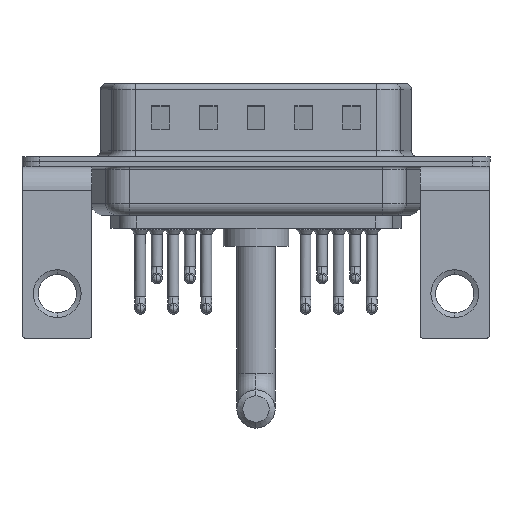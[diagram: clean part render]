
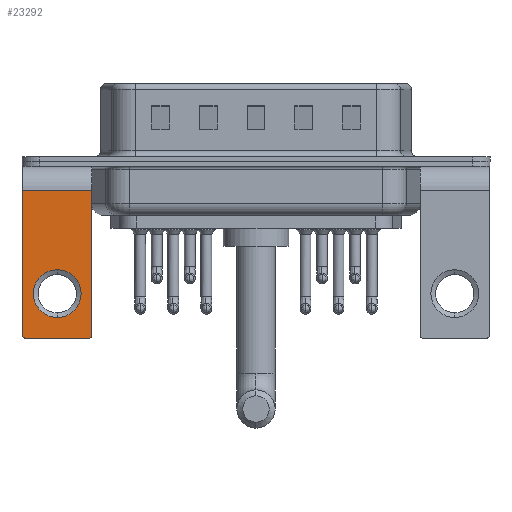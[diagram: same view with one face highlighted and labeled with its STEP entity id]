
A CAD part, front view. The second image highlights one B-rep face of the part: STEP entity #23292.
In plain terms, the highlighted planar face has unit normal (0, -1, 0).
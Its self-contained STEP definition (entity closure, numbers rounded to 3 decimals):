
#25 = CIRCLE ( 'NONE', #10216, 0.25 ) ;
#61 = VERTEX_POINT ( 'NONE', #17904 ) ;
#347 = CIRCLE ( 'NONE', #19550, 0.25 ) ;
#597 = ORIENTED_EDGE ( 'NONE', *, *, #881, .T. ) ;
#718 = VECTOR ( 'NONE', #18286, 1000. ) ;
#881 = EDGE_CURVE ( 'NONE', #8379, #8032, #25, .T. ) ;
#1021 = EDGE_CURVE ( 'NONE', #61, #8032, #4256, .T. ) ;
#1124 = CARTESIAN_POINT ( 'NONE',  ( 2.65, -6.25, -14.55 ) ) ;
#1234 = AXIS2_PLACEMENT_3D ( 'NONE', #17375, #6524, #15369 ) ;
#1871 = VECTOR ( 'NONE', #6179, 1000. ) ;
#1975 = CIRCLE ( 'NONE', #1234, 2. ) ;
#2732 = CARTESIAN_POINT ( 'NONE',  ( 0., -6.25, -9.07 ) ) ;
#3283 = CARTESIAN_POINT ( 'NONE',  ( 2.9, -6.25, -14.55 ) ) ;
#3913 = DIRECTION ( 'NONE',  ( 0., 0., 1. ) ) ;
#4009 = ORIENTED_EDGE ( 'NONE', *, *, #1021, .F. ) ;
#4030 = FACE_BOUND ( 'NONE', #14153, .T. ) ;
#4256 = LINE ( 'NONE', #13473, #19244 ) ;
#4351 = VERTEX_POINT ( 'NONE', #13521 ) ;
#4848 = CARTESIAN_POINT ( 'NONE',  ( 2.9, -6.25, -2.4 ) ) ;
#5920 = EDGE_CURVE ( 'NONE', #21514, #14143, #18168, .T. ) ;
#6023 = EDGE_CURVE ( 'NONE', #14143, #4351, #347, .T. ) ;
#6179 = DIRECTION ( 'NONE',  ( -1., 0., 0. ) ) ;
#6257 = ORIENTED_EDGE ( 'NONE', *, *, #6023, .T. ) ;
#6524 = DIRECTION ( 'NONE',  ( 0., 1., 0. ) ) ;
#6942 = AXIS2_PLACEMENT_3D ( 'NONE', #18237, #18593, #9760 ) ;
#6956 = VERTEX_POINT ( 'NONE', #22249 ) ;
#7449 = CARTESIAN_POINT ( 'NONE',  ( -2.9, -6.25, -2.4 ) ) ;
#7915 = ORIENTED_EDGE ( 'NONE', *, *, #5920, .T. ) ;
#8032 = VERTEX_POINT ( 'NONE', #3283 ) ;
#8379 = VERTEX_POINT ( 'NONE', #22612 ) ;
#8402 = ORIENTED_EDGE ( 'NONE', *, *, #19854, .T. ) ;
#9491 = EDGE_CURVE ( 'NONE', #16404, #6956, #17115, .T. ) ;
#9532 = ORIENTED_EDGE ( 'NONE', *, *, #20257, .T. ) ;
#9760 = DIRECTION ( 'NONE',  ( 0., 0., 1. ) ) ;
#9803 = LINE ( 'NONE', #4848, #22710 ) ;
#10216 = AXIS2_PLACEMENT_3D ( 'NONE', #1124, #15621, #21278 ) ;
#11228 = PLANE ( 'NONE',  #11857 ) ;
#11342 = CARTESIAN_POINT ( 'NONE',  ( -2.9, -6.25, -2.4 ) ) ;
#11343 = DIRECTION ( 'NONE',  ( 0., 0., 1. ) ) ;
#11497 = LINE ( 'NONE', #17154, #1871 ) ;
#11595 = ORIENTED_EDGE ( 'NONE', *, *, #9491, .T. ) ;
#11857 = AXIS2_PLACEMENT_3D ( 'NONE', #12543, #20061, #3913 ) ;
#12543 = CARTESIAN_POINT ( 'NONE',  ( 2.9, -6.25, -2.4 ) ) ;
#13473 = CARTESIAN_POINT ( 'NONE',  ( 2.9, -6.25, -2.4 ) ) ;
#13521 = CARTESIAN_POINT ( 'NONE',  ( -2.65, -6.25, -14.8 ) ) ;
#13810 = DIRECTION ( 'NONE',  ( -1., 0., 0. ) ) ;
#14143 = VERTEX_POINT ( 'NONE', #16857 ) ;
#14153 = EDGE_LOOP ( 'NONE', ( #8402, #11595 ) ) ;
#14746 = EDGE_LOOP ( 'NONE', ( #7915, #6257, #20436, #597, #4009, #9532 ) ) ;
#15369 = DIRECTION ( 'NONE',  ( 0., 0., 1. ) ) ;
#15621 = DIRECTION ( 'NONE',  ( 0., -1., 0. ) ) ;
#15919 = EDGE_CURVE ( 'NONE', #8379, #4351, #11497, .T. ) ;
#16404 = VERTEX_POINT ( 'NONE', #2732 ) ;
#16646 = FACE_OUTER_BOUND ( 'NONE', #14746, .T. ) ;
#16857 = CARTESIAN_POINT ( 'NONE',  ( -2.9, -6.25, -14.55 ) ) ;
#17115 = CIRCLE ( 'NONE', #6942, 2. ) ;
#17154 = CARTESIAN_POINT ( 'NONE',  ( 2.9, -6.25, -14.8 ) ) ;
#17375 = CARTESIAN_POINT ( 'NONE',  ( 0., -6.25, -11.07 ) ) ;
#17904 = CARTESIAN_POINT ( 'NONE',  ( 2.9, -6.25, -2.4 ) ) ;
#18168 = LINE ( 'NONE', #7449, #718 ) ;
#18237 = CARTESIAN_POINT ( 'NONE',  ( 0., -6.25, -11.07 ) ) ;
#18286 = DIRECTION ( 'NONE',  ( 0., 0., -1. ) ) ;
#18400 = CARTESIAN_POINT ( 'NONE',  ( -2.65, -6.25, -14.55 ) ) ;
#18593 = DIRECTION ( 'NONE',  ( 0., 1., 0. ) ) ;
#19244 = VECTOR ( 'NONE', #20537, 1000. ) ;
#19550 = AXIS2_PLACEMENT_3D ( 'NONE', #18400, #21952, #11343 ) ;
#19854 = EDGE_CURVE ( 'NONE', #6956, #16404, #1975, .T. ) ;
#20061 = DIRECTION ( 'NONE',  ( 0., 1., 0. ) ) ;
#20257 = EDGE_CURVE ( 'NONE', #61, #21514, #9803, .T. ) ;
#20436 = ORIENTED_EDGE ( 'NONE', *, *, #15919, .F. ) ;
#20537 = DIRECTION ( 'NONE',  ( 0., 0., -1. ) ) ;
#21278 = DIRECTION ( 'NONE',  ( 0., 0., 1. ) ) ;
#21514 = VERTEX_POINT ( 'NONE', #11342 ) ;
#21952 = DIRECTION ( 'NONE',  ( 0., -1., 0. ) ) ;
#22249 = CARTESIAN_POINT ( 'NONE',  ( 0., -6.25, -13.07 ) ) ;
#22612 = CARTESIAN_POINT ( 'NONE',  ( 2.65, -6.25, -14.8 ) ) ;
#22710 = VECTOR ( 'NONE', #13810, 1000. ) ;
#23292 = ADVANCED_FACE ( 'NONE', ( #4030, #16646 ), #11228, .F. ) ;
